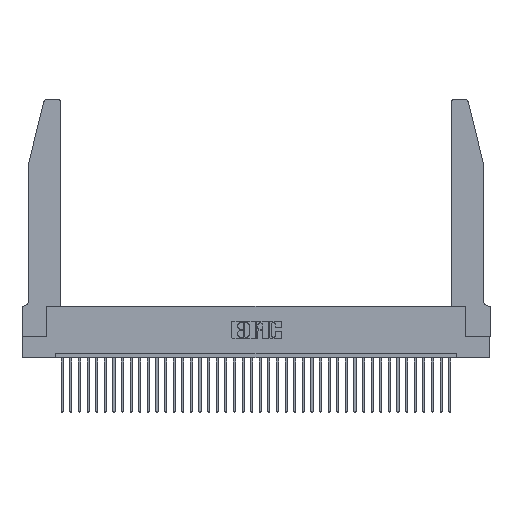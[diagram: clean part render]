
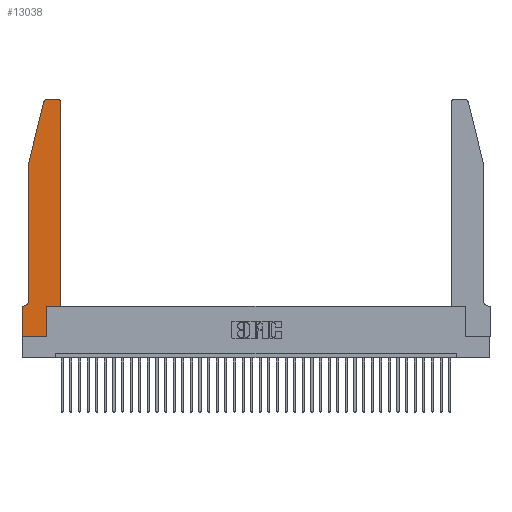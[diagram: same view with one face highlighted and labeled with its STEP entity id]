
A CAD part, top view. The second image highlights one B-rep face of the part: STEP entity #13038.
In plain terms, the highlighted planar face has unit normal (0, 0, 1).
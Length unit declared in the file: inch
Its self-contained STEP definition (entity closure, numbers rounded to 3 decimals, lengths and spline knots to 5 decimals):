
#376 = ORIENTED_EDGE ( 'NONE', *, *, #26933, .T. ) ;
#490 = VERTEX_POINT ( 'NONE', #11942 ) ;
#1097 = EDGE_CURVE ( 'NONE', #5976, #30769, #11384, .T. ) ;
#1775 = CARTESIAN_POINT ( 'NONE',  ( 0., 0.35, 0.37 ) ) ;
#1923 = DIRECTION ( 'NONE',  ( -1., 0., 0. ) ) ;
#2807 = EDGE_CURVE ( 'NONE', #26236, #4051, #36531, .T. ) ;
#2866 = CARTESIAN_POINT ( 'NONE',  ( 0.4505, 2.72, 0.37 ) ) ;
#2990 = LINE ( 'NONE', #38589, #13834 ) ;
#3605 = VECTOR ( 'NONE', #33067, 39.37008 ) ;
#3968 = VERTEX_POINT ( 'NONE', #14290 ) ;
#4051 = VERTEX_POINT ( 'NONE', #20967 ) ;
#4419 = CARTESIAN_POINT ( 'NONE',  ( 0.2865, 0.35, 0.37 ) ) ;
#4669 = CARTESIAN_POINT ( 'NONE',  ( 0.4505, 0.35, 0.37 ) ) ;
#4786 = DIRECTION ( 'NONE',  ( 1., 0., 0. ) ) ;
#5064 = DIRECTION ( 'NONE',  ( 0., 0., 1. ) ) ;
#5294 = AXIS2_PLACEMENT_3D ( 'NONE', #1775, #5064, #32120 ) ;
#5699 = EDGE_CURVE ( 'NONE', #490, #35571, #31849, .T. ) ;
#5814 = DIRECTION ( 'NONE',  ( 0., 1., 0. ) ) ;
#5976 = VERTEX_POINT ( 'NONE', #28561 ) ;
#6023 = DIRECTION ( 'NONE',  ( 1., 0., 0. ) ) ;
#6322 = ORIENTED_EDGE ( 'NONE', *, *, #33035, .T. ) ;
#6380 = LINE ( 'NONE', #4669, #38329 ) ;
#6442 = VECTOR ( 'NONE', #33870, 39.37008 ) ;
#7198 = VECTOR ( 'NONE', #34353, 39.37008 ) ;
#8215 = ORIENTED_EDGE ( 'NONE', *, *, #5699, .T. ) ;
#8300 = ORIENTED_EDGE ( 'NONE', *, *, #31724, .T. ) ;
#8505 = CARTESIAN_POINT ( 'NONE',  ( 0.0055, 0.35, 0.37 ) ) ;
#9052 = DIRECTION ( 'NONE',  ( 0., 0., 1. ) ) ;
#9152 = DIRECTION ( 'NONE',  ( 0., 0., 1. ) ) ;
#9272 = DIRECTION ( 'NONE',  ( -1., 0., 0. ) ) ;
#10487 = AXIS2_PLACEMENT_3D ( 'NONE', #33161, #9152, #6023 ) ;
#11384 = CIRCLE ( 'NONE', #25107, 0.03 ) ;
#11942 = CARTESIAN_POINT ( 'NONE',  ( 0.2865, 0., 0.37 ) ) ;
#12044 = CARTESIAN_POINT ( 'NONE',  ( 0.0755, 0.35, 0.37 ) ) ;
#12124 = CIRCLE ( 'NONE', #10487, 0.03 ) ;
#12327 = CARTESIAN_POINT ( 'NONE',  ( 0.2865, 0.35, 0.37 ) ) ;
#12362 = ORIENTED_EDGE ( 'NONE', *, *, #34283, .T. ) ;
#12664 = CARTESIAN_POINT ( 'NONE',  ( 0.4505, 0.35, 0.37 ) ) ;
#12848 = LINE ( 'NONE', #13091, #7198 ) ;
#13038 = ADVANCED_FACE ( 'NONE', ( #26148 ), #22966, .T. ) ;
#13091 = CARTESIAN_POINT ( 'NONE',  ( 0.0755, 2., 0.37 ) ) ;
#13834 = VECTOR ( 'NONE', #5814, 39.37008 ) ;
#13962 = VERTEX_POINT ( 'NONE', #8505 ) ;
#14290 = CARTESIAN_POINT ( 'NONE',  ( 0.0755, 2., 0.37 ) ) ;
#14521 = CARTESIAN_POINT ( 'NONE',  ( 0., 0., 0.37 ) ) ;
#15552 = CIRCLE ( 'NONE', #36559, 0.07 ) ;
#15566 = CARTESIAN_POINT ( 'NONE',  ( 0.0755, 0.42, 0.37 ) ) ;
#17346 = LINE ( 'NONE', #36175, #37939 ) ;
#17750 = EDGE_CURVE ( 'NONE', #4051, #490, #31353, .T. ) ;
#18116 = ORIENTED_EDGE ( 'NONE', *, *, #20826, .T. ) ;
#19187 = VERTEX_POINT ( 'NONE', #34134 ) ;
#19382 = CARTESIAN_POINT ( 'NONE',  ( 0.0755, 2., 0.37 ) ) ;
#19883 = ORIENTED_EDGE ( 'NONE', *, *, #35018, .T. ) ;
#20144 = ORIENTED_EDGE ( 'NONE', *, *, #1097, .T. ) ;
#20297 = LINE ( 'NONE', #19382, #35305 ) ;
#20826 = EDGE_CURVE ( 'NONE', #3968, #24985, #20297, .T. ) ;
#20967 = CARTESIAN_POINT ( 'NONE',  ( 0., 0., 0.37 ) ) ;
#22634 = EDGE_CURVE ( 'NONE', #19187, #5976, #17346, .T. ) ;
#22966 = PLANE ( 'NONE',  #5294 ) ;
#23422 = VECTOR ( 'NONE', #31058, 39.37008 ) ;
#23474 = CARTESIAN_POINT ( 'NONE',  ( 0.25487, 2.72718, 0.37 ) ) ;
#23534 = CARTESIAN_POINT ( 'NONE',  ( 0.0055, 0.42, 0.37 ) ) ;
#23895 = LINE ( 'NONE', #12044, #3605 ) ;
#24007 = ORIENTED_EDGE ( 'NONE', *, *, #22634, .T. ) ;
#24985 = VERTEX_POINT ( 'NONE', #15566 ) ;
#25107 = AXIS2_PLACEMENT_3D ( 'NONE', #27274, #9052, #4786 ) ;
#25132 = ORIENTED_EDGE ( 'NONE', *, *, #36278, .T. ) ;
#26148 = FACE_OUTER_BOUND ( 'NONE', #28801, .T. ) ;
#26236 = VERTEX_POINT ( 'NONE', #36702 ) ;
#26307 = VECTOR ( 'NONE', #29611, 39.37008 ) ;
#26933 = EDGE_CURVE ( 'NONE', #31486, #37240, #2990, .T. ) ;
#27274 = CARTESIAN_POINT ( 'NONE',  ( 0.284, 2.72, 0.37 ) ) ;
#27874 = CARTESIAN_POINT ( 'NONE',  ( 0., 0., 0.37 ) ) ;
#28561 = CARTESIAN_POINT ( 'NONE',  ( 0.284, 2.75, 0.37 ) ) ;
#28801 = EDGE_LOOP ( 'NONE', ( #24007, #20144, #25132, #18116, #8300, #12362, #34186, #36931, #8215, #19883, #376, #6322 ) ) ;
#29395 = DIRECTION ( 'NONE',  ( 0., 0., -1. ) ) ;
#29611 = DIRECTION ( 'NONE',  ( 0., -1., 0. ) ) ;
#30769 = VERTEX_POINT ( 'NONE', #23474 ) ;
#31058 = DIRECTION ( 'NONE',  ( 0., 1., 0. ) ) ;
#31353 = LINE ( 'NONE', #27874, #6442 ) ;
#31486 = VERTEX_POINT ( 'NONE', #12664 ) ;
#31724 = EDGE_CURVE ( 'NONE', #24985, #13962, #15552, .T. ) ;
#31849 = LINE ( 'NONE', #4419, #23422 ) ;
#32120 = DIRECTION ( 'NONE',  ( 1., 0., 0. ) ) ;
#33035 = EDGE_CURVE ( 'NONE', #37240, #19187, #12124, .T. ) ;
#33067 = DIRECTION ( 'NONE',  ( -1., 0., 0. ) ) ;
#33161 = CARTESIAN_POINT ( 'NONE',  ( 0.4205, 2.72, 0.37 ) ) ;
#33870 = DIRECTION ( 'NONE',  ( 1., 0., 0. ) ) ;
#34134 = CARTESIAN_POINT ( 'NONE',  ( 0.4205, 2.75, 0.37 ) ) ;
#34186 = ORIENTED_EDGE ( 'NONE', *, *, #2807, .T. ) ;
#34283 = EDGE_CURVE ( 'NONE', #13962, #26236, #23895, .T. ) ;
#34353 = DIRECTION ( 'NONE',  ( -0.239, -0.971, 0. ) ) ;
#35018 = EDGE_CURVE ( 'NONE', #35571, #31486, #6380, .T. ) ;
#35305 = VECTOR ( 'NONE', #37319, 39.37008 ) ;
#35571 = VERTEX_POINT ( 'NONE', #12327 ) ;
#36175 = CARTESIAN_POINT ( 'NONE',  ( 0.2605, 2.75, 0.37 ) ) ;
#36278 = EDGE_CURVE ( 'NONE', #30769, #3968, #12848, .T. ) ;
#36531 = LINE ( 'NONE', #14521, #26307 ) ;
#36559 = AXIS2_PLACEMENT_3D ( 'NONE', #23534, #29395, #1923 ) ;
#36702 = CARTESIAN_POINT ( 'NONE',  ( 0., 0.35, 0.37 ) ) ;
#36931 = ORIENTED_EDGE ( 'NONE', *, *, #17750, .T. ) ;
#37051 = DIRECTION ( 'NONE',  ( 1., 0., 0. ) ) ;
#37240 = VERTEX_POINT ( 'NONE', #2866 ) ;
#37319 = DIRECTION ( 'NONE',  ( 0., -1., 0. ) ) ;
#37939 = VECTOR ( 'NONE', #9272, 39.37008 ) ;
#38329 = VECTOR ( 'NONE', #37051, 39.37008 ) ;
#38589 = CARTESIAN_POINT ( 'NONE',  ( 0.4505, 0.35, 0.37 ) ) ;
